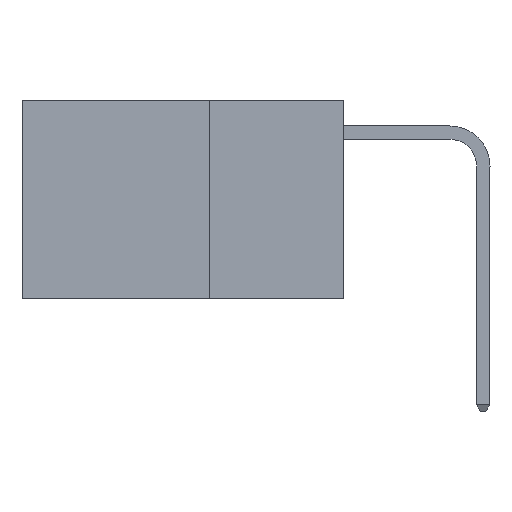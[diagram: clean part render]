
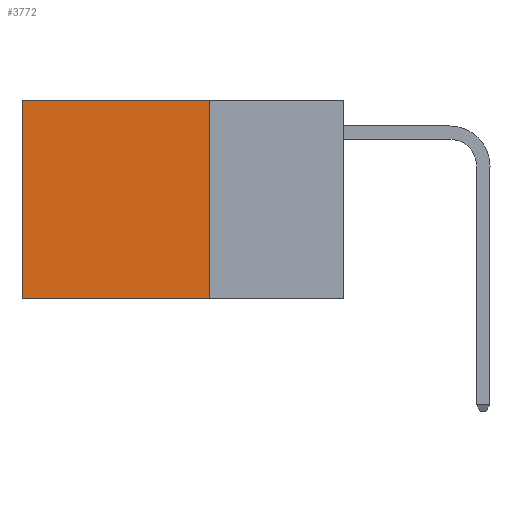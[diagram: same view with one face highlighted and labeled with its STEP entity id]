
A CAD part, left-side view. The second image highlights one B-rep face of the part: STEP entity #3772.
In plain terms, the highlighted planar face has unit normal (-1, 0, 0).
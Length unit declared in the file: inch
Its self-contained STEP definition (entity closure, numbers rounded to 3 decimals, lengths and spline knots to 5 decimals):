
#145 = VECTOR ( 'NONE', #898, 39.37008 ) ;
#530 = DIRECTION ( 'NONE',  ( 0., 1., 0. ) ) ;
#898 = DIRECTION ( 'NONE',  ( 0., 1., 0. ) ) ;
#1248 = DIRECTION ( 'NONE',  ( 0., 0., -1. ) ) ;
#1268 = DIRECTION ( 'NONE',  ( 1., 0., 0. ) ) ;
#1286 = PLANE ( 'NONE',  #12549 ) ;
#1337 = CARTESIAN_POINT ( 'NONE',  ( 0.2625, 0.25, 0. ) ) ;
#2625 = DIRECTION ( 'NONE',  ( 0., 0., -1. ) ) ;
#2939 = LINE ( 'NONE', #4925, #12026 ) ;
#2981 = CARTESIAN_POINT ( 'NONE',  ( 0.2625, 0.25, 0. ) ) ;
#3772 = ADVANCED_FACE ( 'NONE', ( #9954 ), #1286, .F. ) ;
#3874 = CARTESIAN_POINT ( 'NONE',  ( 0.2625, 0.25, 0. ) ) ;
#4925 = CARTESIAN_POINT ( 'NONE',  ( 0.2625, 0.6, 0. ) ) ;
#4944 = ORIENTED_EDGE ( 'NONE', *, *, #10212, .F. ) ;
#5028 = VERTEX_POINT ( 'NONE', #5039 ) ;
#5039 = CARTESIAN_POINT ( 'NONE',  ( 0.2625, 0.25, 0. ) ) ;
#5251 = EDGE_CURVE ( 'NONE', #5028, #9860, #5552, .T. ) ;
#5290 = VERTEX_POINT ( 'NONE', #15363 ) ;
#5469 = LINE ( 'NONE', #3874, #8400 ) ;
#5552 = LINE ( 'NONE', #2981, #11759 ) ;
#5614 = EDGE_LOOP ( 'NONE', ( #6022, #4944, #13244, #14362 ) ) ;
#6022 = ORIENTED_EDGE ( 'NONE', *, *, #8365, .T. ) ;
#7836 = VERTEX_POINT ( 'NONE', #10135 ) ;
#8352 = CARTESIAN_POINT ( 'NONE',  ( 0.2625, 0.25, -0.37 ) ) ;
#8365 = EDGE_CURVE ( 'NONE', #9860, #7836, #2939, .T. ) ;
#8400 = VECTOR ( 'NONE', #2625, 39.37008 ) ;
#9649 = LINE ( 'NONE', #8352, #145 ) ;
#9860 = VERTEX_POINT ( 'NONE', #10123 ) ;
#9954 = FACE_OUTER_BOUND ( 'NONE', #5614, .T. ) ;
#10123 = CARTESIAN_POINT ( 'NONE',  ( 0.2625, 0.6, 0. ) ) ;
#10135 = CARTESIAN_POINT ( 'NONE',  ( 0.2625, 0.6, -0.37 ) ) ;
#10212 = EDGE_CURVE ( 'NONE', #5290, #7836, #9649, .T. ) ;
#11086 = DIRECTION ( 'NONE',  ( 0., 0., -1. ) ) ;
#11759 = VECTOR ( 'NONE', #530, 39.37008 ) ;
#12026 = VECTOR ( 'NONE', #11086, 39.37008 ) ;
#12302 = EDGE_CURVE ( 'NONE', #5028, #5290, #5469, .T. ) ;
#12549 = AXIS2_PLACEMENT_3D ( 'NONE', #1337, #1268, #1248 ) ;
#13244 = ORIENTED_EDGE ( 'NONE', *, *, #12302, .F. ) ;
#14362 = ORIENTED_EDGE ( 'NONE', *, *, #5251, .T. ) ;
#15363 = CARTESIAN_POINT ( 'NONE',  ( 0.2625, 0.25, -0.37 ) ) ;
